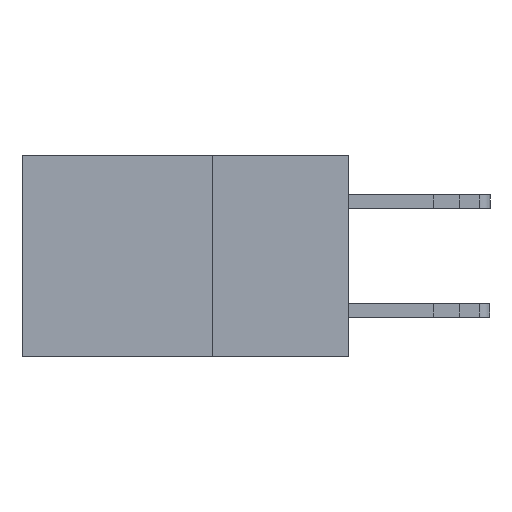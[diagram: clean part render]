
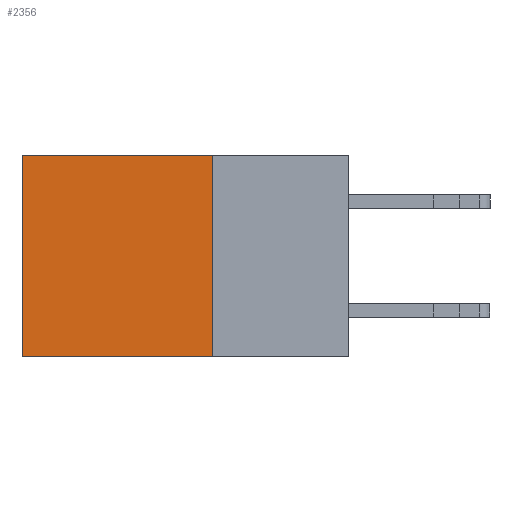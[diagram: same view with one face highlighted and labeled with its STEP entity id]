
A CAD part, left-side view. The second image highlights one B-rep face of the part: STEP entity #2356.
In plain terms, the highlighted planar face has unit normal (-1, 0, 0).
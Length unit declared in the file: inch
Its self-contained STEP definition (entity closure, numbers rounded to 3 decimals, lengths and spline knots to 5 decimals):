
#91 = CARTESIAN_POINT ( 'NONE',  ( 0.298, 0.25, 0. ) ) ;
#380 = CARTESIAN_POINT ( 'NONE',  ( 0.298, 0.6, -0.37 ) ) ;
#591 = CARTESIAN_POINT ( 'NONE',  ( 0.298, 0.25, -0.37 ) ) ;
#1066 = CARTESIAN_POINT ( 'NONE',  ( 0.298, 0.25, -0.37 ) ) ;
#1693 = PLANE ( 'NONE',  #4925 ) ;
#1817 = DIRECTION ( 'NONE',  ( 1., 0., 0. ) ) ;
#2356 = ADVANCED_FACE ( 'NONE', ( #14495 ), #1693, .F. ) ;
#3592 = EDGE_CURVE ( 'NONE', #12829, #4225, #12198, .T. ) ;
#4225 = VERTEX_POINT ( 'NONE', #380 ) ;
#4631 = DIRECTION ( 'NONE',  ( 0., 1., 0. ) ) ;
#4925 = AXIS2_PLACEMENT_3D ( 'NONE', #91, #1817, #10879 ) ;
#4969 = LINE ( 'NONE', #16629, #11290 ) ;
#5807 = EDGE_CURVE ( 'NONE', #16254, #12829, #4969, .T. ) ;
#6376 = VECTOR ( 'NONE', #10517, 39.37008 ) ;
#6865 = EDGE_LOOP ( 'NONE', ( #9201, #7966, #15616, #16262 ) ) ;
#7966 = ORIENTED_EDGE ( 'NONE', *, *, #16559, .F. ) ;
#8241 = CARTESIAN_POINT ( 'NONE',  ( 0.298, 0.6, 0. ) ) ;
#8400 = VECTOR ( 'NONE', #8565, 39.37008 ) ;
#8565 = DIRECTION ( 'NONE',  ( 0., 1., 0. ) ) ;
#8617 = VECTOR ( 'NONE', #15238, 39.37008 ) ;
#9147 = CARTESIAN_POINT ( 'NONE',  ( 0.298, 0.25, 0. ) ) ;
#9201 = ORIENTED_EDGE ( 'NONE', *, *, #3592, .T. ) ;
#9279 = CARTESIAN_POINT ( 'NONE',  ( 0.298, 0.25, 0. ) ) ;
#10366 = LINE ( 'NONE', #9147, #6376 ) ;
#10517 = DIRECTION ( 'NONE',  ( 0., 0., -1. ) ) ;
#10879 = DIRECTION ( 'NONE',  ( 0., 0., -1. ) ) ;
#11290 = VECTOR ( 'NONE', #4631, 39.37008 ) ;
#11431 = CARTESIAN_POINT ( 'NONE',  ( 0.298, 0.6, 0. ) ) ;
#12198 = LINE ( 'NONE', #11431, #8617 ) ;
#12829 = VERTEX_POINT ( 'NONE', #8241 ) ;
#14495 = FACE_OUTER_BOUND ( 'NONE', #6865, .T. ) ;
#15057 = EDGE_CURVE ( 'NONE', #16254, #16787, #10366, .T. ) ;
#15238 = DIRECTION ( 'NONE',  ( 0., 0., -1. ) ) ;
#15407 = LINE ( 'NONE', #591, #8400 ) ;
#15616 = ORIENTED_EDGE ( 'NONE', *, *, #15057, .F. ) ;
#16254 = VERTEX_POINT ( 'NONE', #9279 ) ;
#16262 = ORIENTED_EDGE ( 'NONE', *, *, #5807, .T. ) ;
#16559 = EDGE_CURVE ( 'NONE', #16787, #4225, #15407, .T. ) ;
#16629 = CARTESIAN_POINT ( 'NONE',  ( 0.298, 0.25, 0. ) ) ;
#16787 = VERTEX_POINT ( 'NONE', #1066 ) ;
